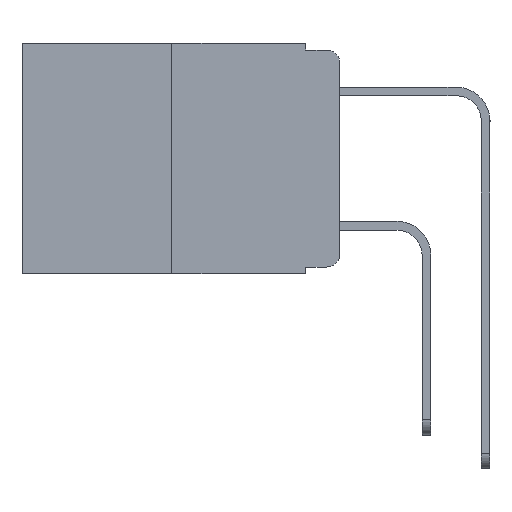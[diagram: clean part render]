
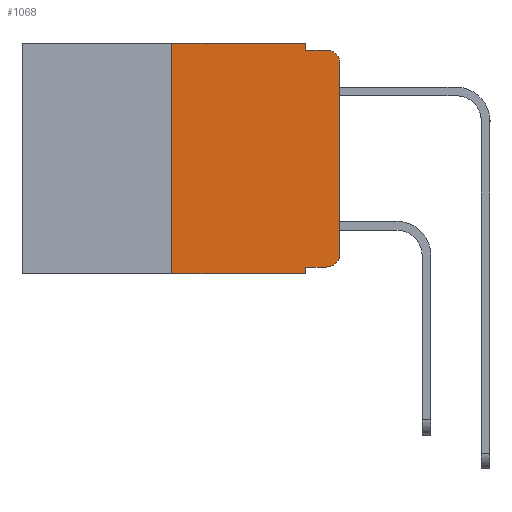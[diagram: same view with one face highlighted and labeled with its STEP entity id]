
A CAD part, left-side view. The second image highlights one B-rep face of the part: STEP entity #1068.
In plain terms, the highlighted planar face has unit normal (-1, 0, 0).
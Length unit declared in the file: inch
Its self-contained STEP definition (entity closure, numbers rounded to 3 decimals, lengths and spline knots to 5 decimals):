
#186 = VERTEX_POINT ( 'NONE', #5414 ) ;
#332 = VERTEX_POINT ( 'NONE', #13774 ) ;
#386 = DIRECTION ( 'NONE',  ( 0., 0., -1. ) ) ;
#525 = VERTEX_POINT ( 'NONE', #8511 ) ;
#694 = VECTOR ( 'NONE', #7352, 39.37008 ) ;
#733 = EDGE_CURVE ( 'NONE', #186, #1347, #9329, .T. ) ;
#839 = DIRECTION ( 'NONE',  ( 0., 0., 1. ) ) ;
#1068 = ADVANCED_FACE ( 'NONE', ( #2130 ), #1857, .F. ) ;
#1286 = LINE ( 'NONE', #3801, #6781 ) ;
#1344 = LINE ( 'NONE', #6398, #4030 ) ;
#1347 = VERTEX_POINT ( 'NONE', #1348 ) ;
#1348 = CARTESIAN_POINT ( 'NONE',  ( 0., 0.051, -0.343 ) ) ;
#1465 = CIRCLE ( 'NONE', #8116, 0.02 ) ;
#1536 = VECTOR ( 'NONE', #5368, 39.37008 ) ;
#1791 = VERTEX_POINT ( 'NONE', #3171 ) ;
#1857 = PLANE ( 'NONE',  #5991 ) ;
#2130 = FACE_OUTER_BOUND ( 'NONE', #13275, .T. ) ;
#2251 = VERTEX_POINT ( 'NONE', #8600 ) ;
#2418 = LINE ( 'NONE', #8471, #5369 ) ;
#2561 = LINE ( 'NONE', #8204, #13369 ) ;
#2575 = EDGE_CURVE ( 'NONE', #8041, #5115, #12455, .T. ) ;
#2620 = ORIENTED_EDGE ( 'NONE', *, *, #11216, .T. ) ;
#2770 = EDGE_CURVE ( 'NONE', #1791, #8530, #1344, .T. ) ;
#3171 = CARTESIAN_POINT ( 'NONE',  ( 0., 0., -0.313 ) ) ;
#3363 = CARTESIAN_POINT ( 'NONE',  ( 0., 0.051, 0. ) ) ;
#3801 = CARTESIAN_POINT ( 'NONE',  ( 0., 0.051, -0.01 ) ) ;
#3849 = CARTESIAN_POINT ( 'NONE',  ( 0., 0.051, -0.01 ) ) ;
#3889 = LINE ( 'NONE', #4134, #6392 ) ;
#4030 = VECTOR ( 'NONE', #11873, 39.37008 ) ;
#4134 = CARTESIAN_POINT ( 'NONE',  ( 0., 0.051, -0.333 ) ) ;
#4227 = ORIENTED_EDGE ( 'NONE', *, *, #4974, .F. ) ;
#4974 = EDGE_CURVE ( 'NONE', #186, #8041, #2418, .T. ) ;
#4980 = DIRECTION ( 'NONE',  ( -1., 0., 0. ) ) ;
#5115 = VERTEX_POINT ( 'NONE', #3363 ) ;
#5141 = CARTESIAN_POINT ( 'NONE',  ( 0., 0., -0.03 ) ) ;
#5368 = DIRECTION ( 'NONE',  ( 0., -1., 0. ) ) ;
#5369 = VECTOR ( 'NONE', #839, 39.37008 ) ;
#5414 = CARTESIAN_POINT ( 'NONE',  ( 0., 0.25, -0.343 ) ) ;
#5712 = ORIENTED_EDGE ( 'NONE', *, *, #2575, .F. ) ;
#5991 = AXIS2_PLACEMENT_3D ( 'NONE', #10397, #12416, #12451 ) ;
#6047 = DIRECTION ( 'NONE',  ( 0., 0., -1. ) ) ;
#6392 = VECTOR ( 'NONE', #11349, 39.37008 ) ;
#6398 = CARTESIAN_POINT ( 'NONE',  ( 0., 0., 0. ) ) ;
#6539 = ORIENTED_EDGE ( 'NONE', *, *, #8324, .F. ) ;
#6781 = VECTOR ( 'NONE', #12098, 39.37008 ) ;
#6989 = CARTESIAN_POINT ( 'NONE',  ( 0., 0.473, -0.343 ) ) ;
#7016 = DIRECTION ( 'NONE',  ( -1., 0., 0. ) ) ;
#7019 = ORIENTED_EDGE ( 'NONE', *, *, #7329, .F. ) ;
#7147 = EDGE_CURVE ( 'NONE', #2251, #1791, #1465, .T. ) ;
#7329 = EDGE_CURVE ( 'NONE', #332, #1347, #2561, .T. ) ;
#7352 = DIRECTION ( 'NONE',  ( 0., -1., 0. ) ) ;
#8041 = VERTEX_POINT ( 'NONE', #12791 ) ;
#8116 = AXIS2_PLACEMENT_3D ( 'NONE', #13139, #7016, #386 ) ;
#8204 = CARTESIAN_POINT ( 'NONE',  ( 0., 0.051, 0. ) ) ;
#8324 = EDGE_CURVE ( 'NONE', #8334, #525, #1286, .T. ) ;
#8334 = VERTEX_POINT ( 'NONE', #3849 ) ;
#8417 = VECTOR ( 'NONE', #10695, 39.37008 ) ;
#8471 = CARTESIAN_POINT ( 'NONE',  ( 0., 0.25, 0. ) ) ;
#8511 = CARTESIAN_POINT ( 'NONE',  ( 0., 0.02, -0.01 ) ) ;
#8530 = VERTEX_POINT ( 'NONE', #5141 ) ;
#8600 = CARTESIAN_POINT ( 'NONE',  ( 0., 0.02, -0.333 ) ) ;
#8718 = AXIS2_PLACEMENT_3D ( 'NONE', #11107, #4980, #12155 ) ;
#8725 = CARTESIAN_POINT ( 'NONE',  ( 0., 0.051, 0. ) ) ;
#9329 = LINE ( 'NONE', #6989, #694 ) ;
#9477 = CIRCLE ( 'NONE', #8718, 0.02 ) ;
#10079 = EDGE_CURVE ( 'NONE', #8530, #525, #9477, .T. ) ;
#10397 = CARTESIAN_POINT ( 'NONE',  ( 0., 0.473, 0. ) ) ;
#10678 = CARTESIAN_POINT ( 'NONE',  ( 0., 0.473, 0. ) ) ;
#10683 = ORIENTED_EDGE ( 'NONE', *, *, #10079, .T. ) ;
#10695 = DIRECTION ( 'NONE',  ( 0., 0., -1. ) ) ;
#10698 = ORIENTED_EDGE ( 'NONE', *, *, #733, .T. ) ;
#11107 = CARTESIAN_POINT ( 'NONE',  ( 0., 0.02, -0.03 ) ) ;
#11216 = EDGE_CURVE ( 'NONE', #332, #2251, #3889, .T. ) ;
#11349 = DIRECTION ( 'NONE',  ( 0., -1., 0. ) ) ;
#11873 = DIRECTION ( 'NONE',  ( 0., 0., 1. ) ) ;
#12098 = DIRECTION ( 'NONE',  ( 0., -1., 0. ) ) ;
#12155 = DIRECTION ( 'NONE',  ( 0., 0., -1. ) ) ;
#12293 = ORIENTED_EDGE ( 'NONE', *, *, #7147, .T. ) ;
#12296 = ORIENTED_EDGE ( 'NONE', *, *, #12544, .F. ) ;
#12416 = DIRECTION ( 'NONE',  ( 1., 0., 0. ) ) ;
#12451 = DIRECTION ( 'NONE',  ( 0., 0., -1. ) ) ;
#12455 = LINE ( 'NONE', #10678, #1536 ) ;
#12544 = EDGE_CURVE ( 'NONE', #5115, #8334, #13505, .T. ) ;
#12791 = CARTESIAN_POINT ( 'NONE',  ( 0., 0.25, 0. ) ) ;
#13095 = ORIENTED_EDGE ( 'NONE', *, *, #2770, .T. ) ;
#13139 = CARTESIAN_POINT ( 'NONE',  ( 0., 0.02, -0.313 ) ) ;
#13275 = EDGE_LOOP ( 'NONE', ( #13095, #10683, #6539, #12296, #5712, #4227, #10698, #7019, #2620, #12293 ) ) ;
#13369 = VECTOR ( 'NONE', #6047, 39.37008 ) ;
#13505 = LINE ( 'NONE', #8725, #8417 ) ;
#13774 = CARTESIAN_POINT ( 'NONE',  ( 0., 0.051, -0.333 ) ) ;
